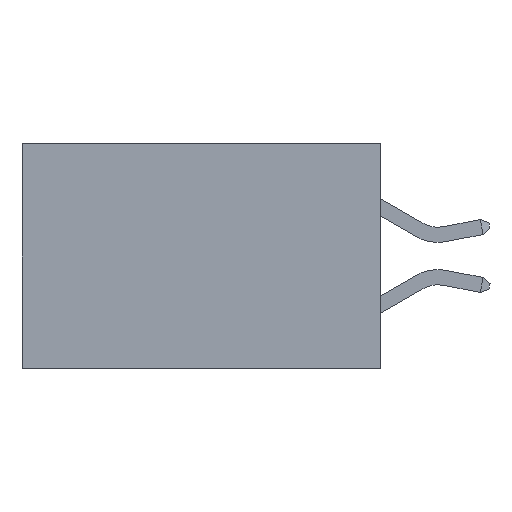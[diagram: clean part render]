
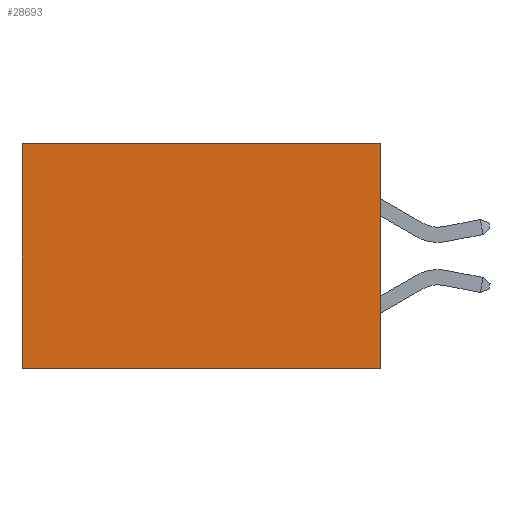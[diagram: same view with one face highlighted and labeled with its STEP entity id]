
A CAD part, left-side view. The second image highlights one B-rep face of the part: STEP entity #28693.
In plain terms, the highlighted planar face has unit normal (-1, 0, 0).
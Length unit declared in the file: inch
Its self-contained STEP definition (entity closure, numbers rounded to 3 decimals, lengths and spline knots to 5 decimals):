
#809 = CARTESIAN_POINT ( 'NONE',  ( 0.277, 0., 0. ) ) ;
#1265 = CARTESIAN_POINT ( 'NONE',  ( 0.277, 0.59, -0.37 ) ) ;
#1679 = CARTESIAN_POINT ( 'NONE',  ( 0.277, 0.59, 0. ) ) ;
#1966 = EDGE_CURVE ( 'NONE', #6682, #3223, #5766, .T. ) ;
#1967 = EDGE_CURVE ( 'NONE', #5267, #32012, #12980, .T. ) ;
#2149 = LINE ( 'NONE', #22505, #9415 ) ;
#3223 = VERTEX_POINT ( 'NONE', #1265 ) ;
#3429 = ORIENTED_EDGE ( 'NONE', *, *, #1966, .F. ) ;
#3553 = ORIENTED_EDGE ( 'NONE', *, *, #4146, .F. ) ;
#3775 = DIRECTION ( 'NONE',  ( 0., 1., 0. ) ) ;
#4146 = EDGE_CURVE ( 'NONE', #5267, #6682, #12421, .T. ) ;
#4851 = ORIENTED_EDGE ( 'NONE', *, *, #1967, .T. ) ;
#5267 = VERTEX_POINT ( 'NONE', #20258 ) ;
#5766 = LINE ( 'NONE', #20928, #33728 ) ;
#6682 = VERTEX_POINT ( 'NONE', #32452 ) ;
#9415 = VECTOR ( 'NONE', #17045, 39.37008 ) ;
#12421 = LINE ( 'NONE', #28490, #25975 ) ;
#12980 = LINE ( 'NONE', #809, #21898 ) ;
#13309 = CARTESIAN_POINT ( 'NONE',  ( 0.277, 0., -0.37 ) ) ;
#17045 = DIRECTION ( 'NONE',  ( 0., 0., -1. ) ) ;
#18653 = PLANE ( 'NONE',  #32750 ) ;
#18766 = DIRECTION ( 'NONE',  ( 0., 0., -1. ) ) ;
#20258 = CARTESIAN_POINT ( 'NONE',  ( 0.277, 0., 0. ) ) ;
#20928 = CARTESIAN_POINT ( 'NONE',  ( 0.277, 0., -0.37 ) ) ;
#20951 = EDGE_CURVE ( 'NONE', #32012, #3223, #2149, .T. ) ;
#21898 = VECTOR ( 'NONE', #3775, 39.37008 ) ;
#22505 = CARTESIAN_POINT ( 'NONE',  ( 0.277, 0.59, -0.37 ) ) ;
#24693 = ORIENTED_EDGE ( 'NONE', *, *, #20951, .T. ) ;
#25975 = VECTOR ( 'NONE', #28191, 39.37008 ) ;
#28191 = DIRECTION ( 'NONE',  ( 0., 0., -1. ) ) ;
#28490 = CARTESIAN_POINT ( 'NONE',  ( 0.277, 0., -0.37 ) ) ;
#28693 = ADVANCED_FACE ( 'NONE', ( #30988 ), #18653, .F. ) ;
#30988 = FACE_OUTER_BOUND ( 'NONE', #31354, .T. ) ;
#31354 = EDGE_LOOP ( 'NONE', ( #24693, #3429, #3553, #4851 ) ) ;
#32012 = VERTEX_POINT ( 'NONE', #1679 ) ;
#32452 = CARTESIAN_POINT ( 'NONE',  ( 0.277, 0., -0.37 ) ) ;
#32750 = AXIS2_PLACEMENT_3D ( 'NONE', #13309, #34945, #18766 ) ;
#33728 = VECTOR ( 'NONE', #33977, 39.37008 ) ;
#33977 = DIRECTION ( 'NONE',  ( 0., 1., 0. ) ) ;
#34945 = DIRECTION ( 'NONE',  ( 1., 0., 0. ) ) ;
